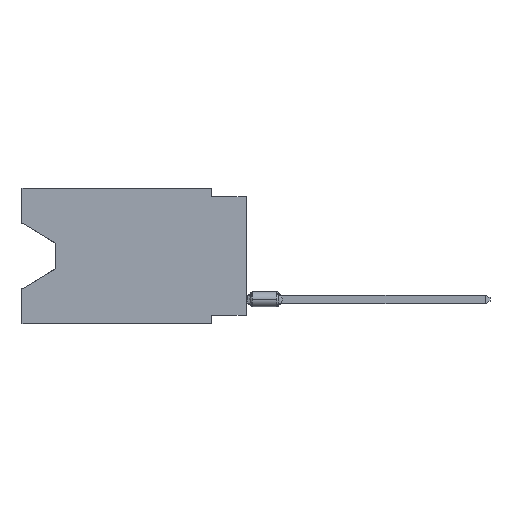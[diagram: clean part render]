
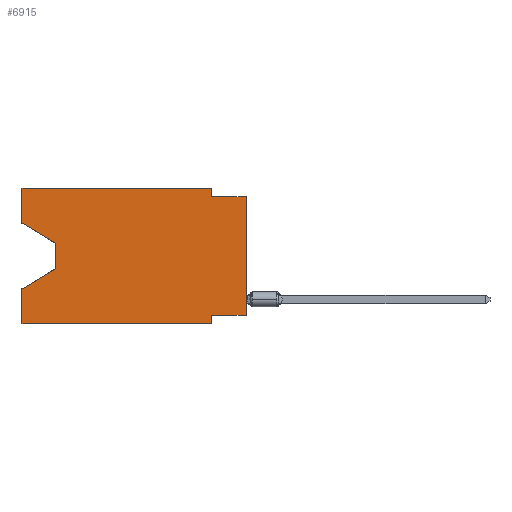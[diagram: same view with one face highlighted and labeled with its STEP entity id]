
A CAD part, left-side view. The second image highlights one B-rep face of the part: STEP entity #6915.
In plain terms, the highlighted planar face has unit normal (-1, 0, 0).
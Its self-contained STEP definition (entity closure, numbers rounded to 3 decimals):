
#4 = DIRECTION ( 'NONE',  ( 0., 1., 0. ) ) ;
#100 = CARTESIAN_POINT ( 'NONE',  ( 0., 16.383, 0. ) ) ;
#361 = CARTESIAN_POINT ( 'NONE',  ( 0., 16.383, -7.36 ) ) ;
#398 = EDGE_CURVE ( 'NONE', #2979, #15300, #8053, .T. ) ;
#538 = CARTESIAN_POINT ( 'NONE',  ( 0., 2.54, 0. ) ) ;
#771 = CARTESIAN_POINT ( 'NONE',  ( 0., 2.54, -9.271 ) ) ;
#832 = DIRECTION ( 'NONE',  ( 0., 0., -1. ) ) ;
#895 = VECTOR ( 'NONE', #5878, 1000. ) ;
#900 = DIRECTION ( 'NONE',  ( 0., 0.855, -0.519 ) ) ;
#1382 = FACE_OUTER_BOUND ( 'NONE', #7600, .T. ) ;
#1446 = ORIENTED_EDGE ( 'NONE', *, *, #9820, .F. ) ;
#1695 = VECTOR ( 'NONE', #4, 1000. ) ;
#1899 = LINE ( 'NONE', #6381, #3287 ) ;
#2192 = VERTEX_POINT ( 'NONE', #771 ) ;
#2326 = LINE ( 'NONE', #538, #12402 ) ;
#2681 = VECTOR ( 'NONE', #7912, 1000. ) ;
#2758 = CARTESIAN_POINT ( 'NONE',  ( 0., 16.383, -9.906 ) ) ;
#2783 = PLANE ( 'NONE',  #7762 ) ;
#2885 = CARTESIAN_POINT ( 'NONE',  ( 0., 16.383, 0. ) ) ;
#2979 = VERTEX_POINT ( 'NONE', #2758 ) ;
#3170 = VECTOR ( 'NONE', #15303, 1000. ) ;
#3287 = VECTOR ( 'NONE', #7681, 1000. ) ;
#3382 = VERTEX_POINT ( 'NONE', #19145 ) ;
#3557 = CARTESIAN_POINT ( 'NONE',  ( 0., 0., -9.271 ) ) ;
#3705 = CARTESIAN_POINT ( 'NONE',  ( 0., 13.97, -4.013 ) ) ;
#3709 = VERTEX_POINT ( 'NONE', #9477 ) ;
#3780 = ORIENTED_EDGE ( 'NONE', *, *, #16696, .F. ) ;
#3994 = EDGE_CURVE ( 'NONE', #7706, #15300, #18823, .T. ) ;
#4223 = CARTESIAN_POINT ( 'NONE',  ( 0., 13.97, -5.893 ) ) ;
#4590 = VECTOR ( 'NONE', #5409, 1000. ) ;
#4681 = LINE ( 'NONE', #7767, #1695 ) ;
#5409 = DIRECTION ( 'NONE',  ( 0., -0.855, -0.519 ) ) ;
#5619 = EDGE_CURVE ( 'NONE', #19656, #3709, #2326, .T. ) ;
#5633 = ORIENTED_EDGE ( 'NONE', *, *, #398, .F. ) ;
#5878 = DIRECTION ( 'NONE',  ( 0., 0., 1. ) ) ;
#6291 = LINE ( 'NONE', #12451, #14429 ) ;
#6301 = EDGE_CURVE ( 'NONE', #12387, #3382, #6590, .T. ) ;
#6381 = CARTESIAN_POINT ( 'NONE',  ( 0., 16.383, 0. ) ) ;
#6590 = LINE ( 'NONE', #15745, #18209 ) ;
#6915 = ADVANCED_FACE ( 'NONE', ( #1382 ), #2783, .F. ) ;
#7072 = ORIENTED_EDGE ( 'NONE', *, *, #10738, .F. ) ;
#7377 = ORIENTED_EDGE ( 'NONE', *, *, #11899, .F. ) ;
#7600 = EDGE_LOOP ( 'NONE', ( #16999, #18980, #12956, #5633, #8771, #7072, #7377, #8969, #14906, #11442, #1446, #3780 ) ) ;
#7632 = CARTESIAN_POINT ( 'NONE',  ( 0., 2.54, 0. ) ) ;
#7681 = DIRECTION ( 'NONE',  ( 0., -1., 0. ) ) ;
#7706 = VERTEX_POINT ( 'NONE', #4223 ) ;
#7762 = AXIS2_PLACEMENT_3D ( 'NONE', #9051, #18294, #15100 ) ;
#7767 = CARTESIAN_POINT ( 'NONE',  ( 0., 0., -9.271 ) ) ;
#7798 = DIRECTION ( 'NONE',  ( 0., 0., -1. ) ) ;
#7912 = DIRECTION ( 'NONE',  ( 0., 0., -1. ) ) ;
#8053 = LINE ( 'NONE', #100, #3170 ) ;
#8234 = CARTESIAN_POINT ( 'NONE',  ( 0., 2.54, -9.906 ) ) ;
#8503 = CARTESIAN_POINT ( 'NONE',  ( 0., 16.383, -2.546 ) ) ;
#8771 = ORIENTED_EDGE ( 'NONE', *, *, #11095, .T. ) ;
#8969 = ORIENTED_EDGE ( 'NONE', *, *, #6301, .T. ) ;
#9051 = CARTESIAN_POINT ( 'NONE',  ( 0., 16.383, 0. ) ) ;
#9410 = CARTESIAN_POINT ( 'NONE',  ( 0., 2.54, -9.906 ) ) ;
#9477 = CARTESIAN_POINT ( 'NONE',  ( 0., 2.54, -0.635 ) ) ;
#9820 = EDGE_CURVE ( 'NONE', #17537, #19656, #1899, .T. ) ;
#10067 = CARTESIAN_POINT ( 'NONE',  ( 0., 13.97, -5.893 ) ) ;
#10090 = CARTESIAN_POINT ( 'NONE',  ( 0., 0., -0.635 ) ) ;
#10738 = EDGE_CURVE ( 'NONE', #2192, #18404, #13868, .T. ) ;
#11095 = EDGE_CURVE ( 'NONE', #2979, #18404, #6291, .T. ) ;
#11162 = VECTOR ( 'NONE', #7798, 1000. ) ;
#11385 = LINE ( 'NONE', #10090, #16624 ) ;
#11401 = VERTEX_POINT ( 'NONE', #16969 ) ;
#11408 = EDGE_CURVE ( 'NONE', #14715, #11401, #13062, .T. ) ;
#11442 = ORIENTED_EDGE ( 'NONE', *, *, #5619, .F. ) ;
#11671 = CARTESIAN_POINT ( 'NONE',  ( 0., 16.383, -2.546 ) ) ;
#11899 = EDGE_CURVE ( 'NONE', #12387, #2192, #4681, .T. ) ;
#12387 = VERTEX_POINT ( 'NONE', #3557 ) ;
#12402 = VECTOR ( 'NONE', #832, 1000. ) ;
#12451 = CARTESIAN_POINT ( 'NONE',  ( 0., 16.383, -9.906 ) ) ;
#12564 = DIRECTION ( 'NONE',  ( 0., 0., 1. ) ) ;
#12711 = VECTOR ( 'NONE', #900, 1000. ) ;
#12956 = ORIENTED_EDGE ( 'NONE', *, *, #3994, .T. ) ;
#13062 = LINE ( 'NONE', #8503, #4590 ) ;
#13868 = LINE ( 'NONE', #9410, #2681 ) ;
#13931 = LINE ( 'NONE', #3705, #11162 ) ;
#14247 = DIRECTION ( 'NONE',  ( 0., -1., 0. ) ) ;
#14429 = VECTOR ( 'NONE', #17123, 1000. ) ;
#14715 = VERTEX_POINT ( 'NONE', #11671 ) ;
#14903 = LINE ( 'NONE', #2885, #895 ) ;
#14906 = ORIENTED_EDGE ( 'NONE', *, *, #16288, .F. ) ;
#15100 = DIRECTION ( 'NONE',  ( 0., 0., -1. ) ) ;
#15300 = VERTEX_POINT ( 'NONE', #361 ) ;
#15303 = DIRECTION ( 'NONE',  ( 0., 0., 1. ) ) ;
#15745 = CARTESIAN_POINT ( 'NONE',  ( 0., 0., 0. ) ) ;
#16288 = EDGE_CURVE ( 'NONE', #3709, #3382, #11385, .T. ) ;
#16624 = VECTOR ( 'NONE', #14247, 1000. ) ;
#16696 = EDGE_CURVE ( 'NONE', #14715, #17537, #14903, .T. ) ;
#16969 = CARTESIAN_POINT ( 'NONE',  ( 0., 13.97, -4.013 ) ) ;
#16999 = ORIENTED_EDGE ( 'NONE', *, *, #11408, .T. ) ;
#17123 = DIRECTION ( 'NONE',  ( 0., -1., 0. ) ) ;
#17128 = CARTESIAN_POINT ( 'NONE',  ( 0., 16.383, 0. ) ) ;
#17537 = VERTEX_POINT ( 'NONE', #17128 ) ;
#17608 = EDGE_CURVE ( 'NONE', #11401, #7706, #13931, .T. ) ;
#18209 = VECTOR ( 'NONE', #12564, 1000. ) ;
#18294 = DIRECTION ( 'NONE',  ( 1., 0., 0. ) ) ;
#18404 = VERTEX_POINT ( 'NONE', #8234 ) ;
#18823 = LINE ( 'NONE', #10067, #12711 ) ;
#18980 = ORIENTED_EDGE ( 'NONE', *, *, #17608, .T. ) ;
#19145 = CARTESIAN_POINT ( 'NONE',  ( 0., 0., -0.635 ) ) ;
#19656 = VERTEX_POINT ( 'NONE', #7632 ) ;
